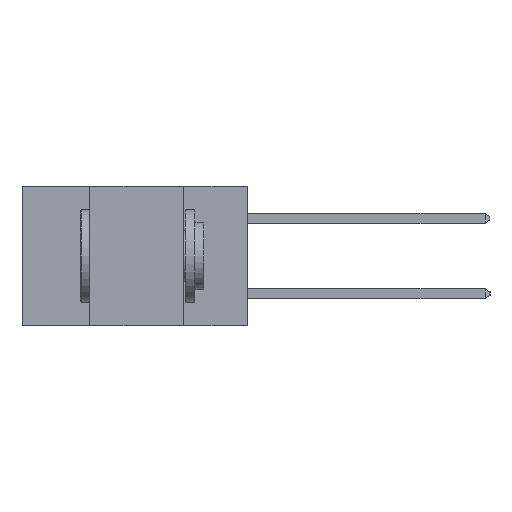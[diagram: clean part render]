
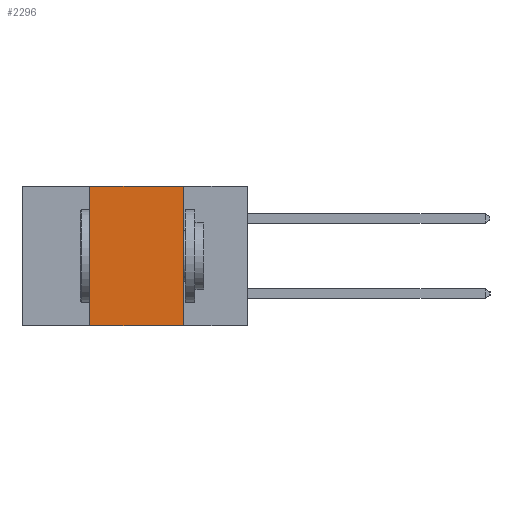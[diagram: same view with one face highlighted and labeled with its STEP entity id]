
A CAD part, left-side view. The second image highlights one B-rep face of the part: STEP entity #2296.
In plain terms, the highlighted planar face has unit normal (-1, 0, 0).
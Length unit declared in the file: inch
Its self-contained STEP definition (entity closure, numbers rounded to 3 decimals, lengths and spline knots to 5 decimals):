
#229 = DIRECTION ( 'NONE',  ( 0., 0., -1. ) ) ;
#538 = VECTOR ( 'NONE', #229, 39.37008 ) ;
#927 = VECTOR ( 'NONE', #7909, 39.37008 ) ;
#929 = AXIS2_PLACEMENT_3D ( 'NONE', #1470, #17362, #17367 ) ;
#931 = DIRECTION ( 'NONE',  ( 0., -1., 0. ) ) ;
#936 = CARTESIAN_POINT ( 'NONE',  ( 0., 0.6, 0. ) ) ;
#1470 = CARTESIAN_POINT ( 'NONE',  ( 0., 0.6, 0. ) ) ;
#2296 = ADVANCED_FACE ( 'NONE', ( #10174 ), #11789, .F. ) ;
#2565 = ORIENTED_EDGE ( 'NONE', *, *, #16760, .T. ) ;
#3239 = VERTEX_POINT ( 'NONE', #12296 ) ;
#3805 = CARTESIAN_POINT ( 'NONE',  ( 0., 0.6, -0.37 ) ) ;
#3856 = LINE ( 'NONE', #936, #14868 ) ;
#4356 = LINE ( 'NONE', #16993, #538 ) ;
#5152 = EDGE_LOOP ( 'NONE', ( #8921, #7425, #5654, #2565 ) ) ;
#5654 = ORIENTED_EDGE ( 'NONE', *, *, #10336, .F. ) ;
#5966 = LINE ( 'NONE', #16118, #12934 ) ;
#7425 = ORIENTED_EDGE ( 'NONE', *, *, #8843, .F. ) ;
#7909 = DIRECTION ( 'NONE',  ( 0., -1., 0. ) ) ;
#8843 = EDGE_CURVE ( 'NONE', #13687, #3239, #3856, .T. ) ;
#8921 = ORIENTED_EDGE ( 'NONE', *, *, #14341, .F. ) ;
#10174 = FACE_OUTER_BOUND ( 'NONE', #5152, .T. ) ;
#10336 = EDGE_CURVE ( 'NONE', #16580, #13687, #5966, .T. ) ;
#11789 = PLANE ( 'NONE',  #929 ) ;
#12296 = CARTESIAN_POINT ( 'NONE',  ( 0., 0.17, 0. ) ) ;
#12934 = VECTOR ( 'NONE', #16077, 39.37008 ) ;
#12999 = VERTEX_POINT ( 'NONE', #15250 ) ;
#13687 = VERTEX_POINT ( 'NONE', #14212 ) ;
#14212 = CARTESIAN_POINT ( 'NONE',  ( 0., 0.42, 0. ) ) ;
#14341 = EDGE_CURVE ( 'NONE', #3239, #12999, #4356, .T. ) ;
#14868 = VECTOR ( 'NONE', #931, 39.37008 ) ;
#15250 = CARTESIAN_POINT ( 'NONE',  ( 0., 0.17, -0.37 ) ) ;
#15769 = LINE ( 'NONE', #3805, #927 ) ;
#15901 = CARTESIAN_POINT ( 'NONE',  ( 0., 0.42, -0.37 ) ) ;
#16077 = DIRECTION ( 'NONE',  ( 0., 0., 1. ) ) ;
#16118 = CARTESIAN_POINT ( 'NONE',  ( 0., 0.42, -0.37 ) ) ;
#16580 = VERTEX_POINT ( 'NONE', #15901 ) ;
#16760 = EDGE_CURVE ( 'NONE', #16580, #12999, #15769, .T. ) ;
#16993 = CARTESIAN_POINT ( 'NONE',  ( 0., 0.17, -0.37 ) ) ;
#17362 = DIRECTION ( 'NONE',  ( 1., 0., 0. ) ) ;
#17367 = DIRECTION ( 'NONE',  ( 0., 0., -1. ) ) ;
